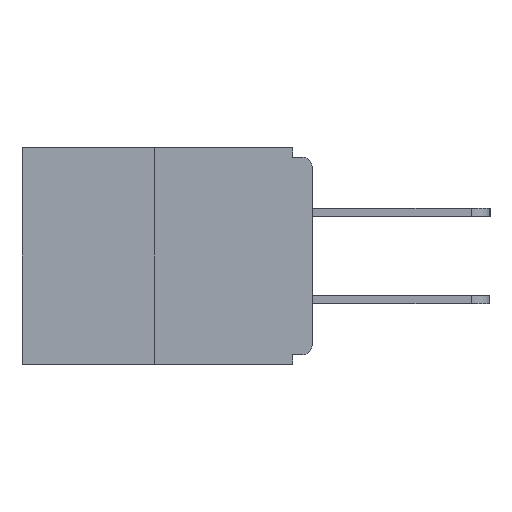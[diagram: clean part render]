
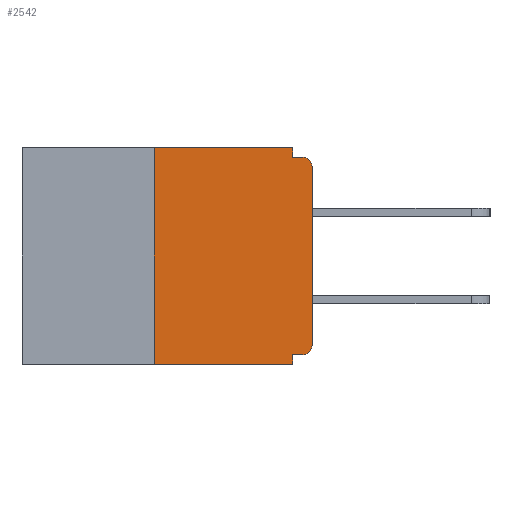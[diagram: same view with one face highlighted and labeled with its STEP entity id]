
A CAD part, left-side view. The second image highlights one B-rep face of the part: STEP entity #2542.
In plain terms, the highlighted planar face has unit normal (-1, 0, 0).
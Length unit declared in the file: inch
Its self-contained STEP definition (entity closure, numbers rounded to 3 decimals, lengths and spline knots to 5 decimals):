
#127 = LINE ( 'NONE', #12379, #12686 ) ;
#280 = CARTESIAN_POINT ( 'NONE',  ( 0., 0.25, -0.343 ) ) ;
#302 = EDGE_CURVE ( 'NONE', #12736, #14523, #901, .T. ) ;
#404 = VERTEX_POINT ( 'NONE', #1088 ) ;
#693 = VECTOR ( 'NONE', #10602, 39.37008 ) ;
#901 = CIRCLE ( 'NONE', #2956, 0.015 ) ;
#1033 = EDGE_CURVE ( 'NONE', #5286, #2422, #9806, .T. ) ;
#1088 = CARTESIAN_POINT ( 'NONE',  ( 0., 0.031, -0.343 ) ) ;
#1143 = DIRECTION ( 'NONE',  ( 0., 0., -1. ) ) ;
#1394 = EDGE_CURVE ( 'NONE', #6012, #404, #7495, .T. ) ;
#1411 = VECTOR ( 'NONE', #1143, 39.37008 ) ;
#1680 = DIRECTION ( 'NONE',  ( 0., 0., -1. ) ) ;
#1722 = VECTOR ( 'NONE', #2457, 39.37008 ) ;
#1880 = EDGE_CURVE ( 'NONE', #14523, #14187, #9988, .T. ) ;
#1949 = CARTESIAN_POINT ( 'NONE',  ( 0., 0., -0.03 ) ) ;
#2279 = AXIS2_PLACEMENT_3D ( 'NONE', #3066, #5520, #1680 ) ;
#2318 = DIRECTION ( 'NONE',  ( 1., 0., 0. ) ) ;
#2422 = VERTEX_POINT ( 'NONE', #13005 ) ;
#2457 = DIRECTION ( 'NONE',  ( 0., -1., 0. ) ) ;
#2542 = ADVANCED_FACE ( 'NONE', ( #10058 ), #13753, .F. ) ;
#2555 = DIRECTION ( 'NONE',  ( 0., 0., 1. ) ) ;
#2626 = CARTESIAN_POINT ( 'NONE',  ( 0., 0.46, 0. ) ) ;
#2956 = AXIS2_PLACEMENT_3D ( 'NONE', #9412, #8281, #5743 ) ;
#3066 = CARTESIAN_POINT ( 'NONE',  ( 0., 0.015, -0.03 ) ) ;
#3723 = LINE ( 'NONE', #7322, #14684 ) ;
#3977 = ORIENTED_EDGE ( 'NONE', *, *, #1033, .F. ) ;
#4336 = CARTESIAN_POINT ( 'NONE',  ( 0., 0.031, 0. ) ) ;
#4921 = CARTESIAN_POINT ( 'NONE',  ( 0., 0., 0. ) ) ;
#5069 = ORIENTED_EDGE ( 'NONE', *, *, #302, .T. ) ;
#5235 = ORIENTED_EDGE ( 'NONE', *, *, #7514, .F. ) ;
#5286 = VERTEX_POINT ( 'NONE', #9982 ) ;
#5476 = EDGE_CURVE ( 'NONE', #2422, #14546, #13095, .T. ) ;
#5520 = DIRECTION ( 'NONE',  ( -1., 0., 0. ) ) ;
#5743 = DIRECTION ( 'NONE',  ( 0., 0., -1. ) ) ;
#5892 = DIRECTION ( 'NONE',  ( 0., 0., -1. ) ) ;
#6012 = VERTEX_POINT ( 'NONE', #15431 ) ;
#6304 = DIRECTION ( 'NONE',  ( 0., -1., 0. ) ) ;
#7043 = EDGE_LOOP ( 'NONE', ( #3977, #5235, #7457, #14706, #14341, #5069, #14478, #11612, #8276, #7260 ) ) ;
#7260 = ORIENTED_EDGE ( 'NONE', *, *, #5476, .F. ) ;
#7322 = CARTESIAN_POINT ( 'NONE',  ( 0., 0.46, -0.343 ) ) ;
#7457 = ORIENTED_EDGE ( 'NONE', *, *, #14352, .T. ) ;
#7495 = LINE ( 'NONE', #14937, #1411 ) ;
#7514 = EDGE_CURVE ( 'NONE', #9025, #5286, #9130, .T. ) ;
#8081 = AXIS2_PLACEMENT_3D ( 'NONE', #2626, #2318, #12451 ) ;
#8276 = ORIENTED_EDGE ( 'NONE', *, *, #8863, .F. ) ;
#8281 = DIRECTION ( 'NONE',  ( -1., 0., 0. ) ) ;
#8486 = VECTOR ( 'NONE', #5892, 39.37008 ) ;
#8715 = DIRECTION ( 'NONE',  ( 0., -1., 0. ) ) ;
#8756 = EDGE_CURVE ( 'NONE', #12736, #6012, #13210, .T. ) ;
#8843 = VECTOR ( 'NONE', #2555, 39.37008 ) ;
#8863 = EDGE_CURVE ( 'NONE', #14546, #8885, #127, .T. ) ;
#8885 = VERTEX_POINT ( 'NONE', #11215 ) ;
#9025 = VERTEX_POINT ( 'NONE', #280 ) ;
#9130 = LINE ( 'NONE', #12904, #693 ) ;
#9412 = CARTESIAN_POINT ( 'NONE',  ( 0., 0.015, -0.313 ) ) ;
#9806 = LINE ( 'NONE', #12356, #1722 ) ;
#9846 = EDGE_CURVE ( 'NONE', #14187, #8885, #16108, .T. ) ;
#9982 = CARTESIAN_POINT ( 'NONE',  ( 0., 0.25, 0. ) ) ;
#9988 = LINE ( 'NONE', #4921, #8843 ) ;
#10058 = FACE_OUTER_BOUND ( 'NONE', #7043, .T. ) ;
#10069 = VECTOR ( 'NONE', #13296, 39.37008 ) ;
#10602 = DIRECTION ( 'NONE',  ( 0., 0., 1. ) ) ;
#11047 = CARTESIAN_POINT ( 'NONE',  ( 0., 0.031, -0.015 ) ) ;
#11215 = CARTESIAN_POINT ( 'NONE',  ( 0., 0.015, -0.015 ) ) ;
#11612 = ORIENTED_EDGE ( 'NONE', *, *, #9846, .T. ) ;
#12356 = CARTESIAN_POINT ( 'NONE',  ( 0., 0.46, 0. ) ) ;
#12379 = CARTESIAN_POINT ( 'NONE',  ( 0., 0., -0.015 ) ) ;
#12451 = DIRECTION ( 'NONE',  ( 0., 0., -1. ) ) ;
#12686 = VECTOR ( 'NONE', #6304, 39.37008 ) ;
#12736 = VERTEX_POINT ( 'NONE', #13931 ) ;
#12904 = CARTESIAN_POINT ( 'NONE',  ( 0., 0.25, 0. ) ) ;
#13005 = CARTESIAN_POINT ( 'NONE',  ( 0., 0.031, 0. ) ) ;
#13095 = LINE ( 'NONE', #4336, #8486 ) ;
#13210 = LINE ( 'NONE', #14504, #10069 ) ;
#13296 = DIRECTION ( 'NONE',  ( 0., 1., 0. ) ) ;
#13753 = PLANE ( 'NONE',  #8081 ) ;
#13931 = CARTESIAN_POINT ( 'NONE',  ( 0., 0.015, -0.328 ) ) ;
#14187 = VERTEX_POINT ( 'NONE', #1949 ) ;
#14341 = ORIENTED_EDGE ( 'NONE', *, *, #8756, .F. ) ;
#14352 = EDGE_CURVE ( 'NONE', #9025, #404, #3723, .T. ) ;
#14478 = ORIENTED_EDGE ( 'NONE', *, *, #1880, .T. ) ;
#14504 = CARTESIAN_POINT ( 'NONE',  ( 0., 0., -0.328 ) ) ;
#14523 = VERTEX_POINT ( 'NONE', #15476 ) ;
#14546 = VERTEX_POINT ( 'NONE', #11047 ) ;
#14684 = VECTOR ( 'NONE', #8715, 39.37008 ) ;
#14706 = ORIENTED_EDGE ( 'NONE', *, *, #1394, .F. ) ;
#14937 = CARTESIAN_POINT ( 'NONE',  ( 0., 0.031, -0.343 ) ) ;
#15431 = CARTESIAN_POINT ( 'NONE',  ( 0., 0.031, -0.328 ) ) ;
#15476 = CARTESIAN_POINT ( 'NONE',  ( 0., 0., -0.313 ) ) ;
#16108 = CIRCLE ( 'NONE', #2279, 0.015 ) ;
